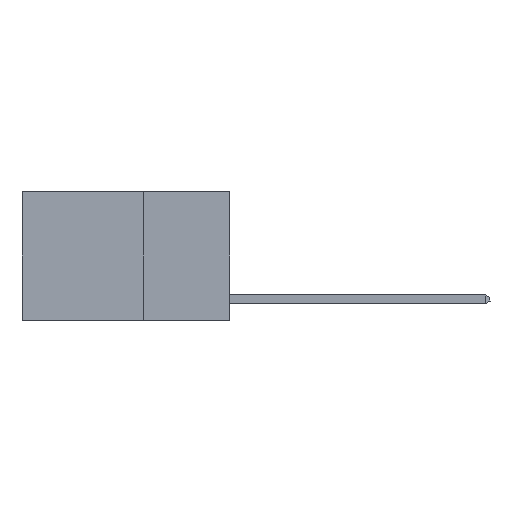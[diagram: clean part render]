
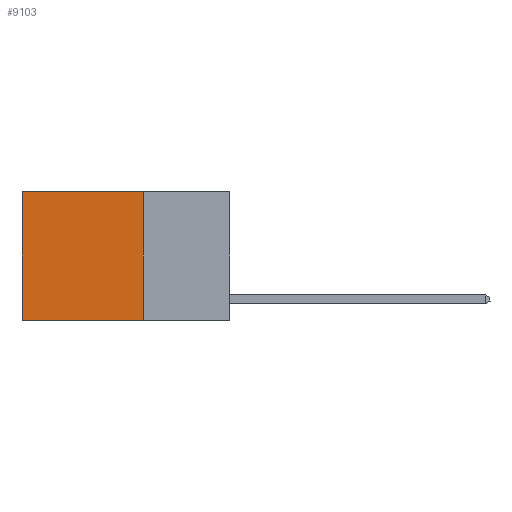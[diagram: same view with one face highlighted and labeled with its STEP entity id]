
A CAD part, left-side view. The second image highlights one B-rep face of the part: STEP entity #9103.
In plain terms, the highlighted planar face has unit normal (-1, 0, 0).
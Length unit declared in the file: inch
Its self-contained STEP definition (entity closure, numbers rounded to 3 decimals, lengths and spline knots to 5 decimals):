
#462 = LINE ( 'NONE', #20775, #28145 ) ;
#796 = ORIENTED_EDGE ( 'NONE', *, *, #27038, .T. ) ;
#2072 = LINE ( 'NONE', #23198, #5950 ) ;
#3762 = AXIS2_PLACEMENT_3D ( 'NONE', #6649, #18120, #24575 ) ;
#4126 = ORIENTED_EDGE ( 'NONE', *, *, #19367, .F. ) ;
#5203 = VECTOR ( 'NONE', #13857, 39.37008 ) ;
#5950 = VECTOR ( 'NONE', #7046, 39.37008 ) ;
#6552 = FACE_OUTER_BOUND ( 'NONE', #15254, .T. ) ;
#6649 = CARTESIAN_POINT ( 'NONE',  ( 0.2625, 0.25, 0. ) ) ;
#7046 = DIRECTION ( 'NONE',  ( 0., 1., 0. ) ) ;
#7233 = EDGE_CURVE ( 'NONE', #23287, #20778, #2072, .T. ) ;
#8322 = EDGE_CURVE ( 'NONE', #26590, #20778, #18528, .T. ) ;
#8589 = CARTESIAN_POINT ( 'NONE',  ( 0.2625, 0.25, 0. ) ) ;
#9103 = ADVANCED_FACE ( 'NONE', ( #6552 ), #14876, .F. ) ;
#11896 = DIRECTION ( 'NONE',  ( 0., 1., 0. ) ) ;
#12887 = LINE ( 'NONE', #8589, #5203 ) ;
#13857 = DIRECTION ( 'NONE',  ( 0., 0., -1. ) ) ;
#14740 = CARTESIAN_POINT ( 'NONE',  ( 0.2625, 0.25, -0.37 ) ) ;
#14876 = PLANE ( 'NONE',  #3762 ) ;
#15254 = EDGE_LOOP ( 'NONE', ( #18761, #21822, #4126, #796 ) ) ;
#15372 = CARTESIAN_POINT ( 'NONE',  ( 0.2625, 0.6, -0.37 ) ) ;
#17946 = CARTESIAN_POINT ( 'NONE',  ( 0.2625, 0.6, 0. ) ) ;
#18120 = DIRECTION ( 'NONE',  ( 1., 0., 0. ) ) ;
#18152 = VECTOR ( 'NONE', #22297, 39.37008 ) ;
#18528 = LINE ( 'NONE', #22395, #18152 ) ;
#18761 = ORIENTED_EDGE ( 'NONE', *, *, #8322, .T. ) ;
#19367 = EDGE_CURVE ( 'NONE', #28267, #23287, #12887, .T. ) ;
#20775 = CARTESIAN_POINT ( 'NONE',  ( 0.2625, 0.25, 0. ) ) ;
#20778 = VERTEX_POINT ( 'NONE', #15372 ) ;
#21822 = ORIENTED_EDGE ( 'NONE', *, *, #7233, .F. ) ;
#22297 = DIRECTION ( 'NONE',  ( 0., 0., -1. ) ) ;
#22395 = CARTESIAN_POINT ( 'NONE',  ( 0.2625, 0.6, 0. ) ) ;
#23198 = CARTESIAN_POINT ( 'NONE',  ( 0.2625, 0.25, -0.37 ) ) ;
#23287 = VERTEX_POINT ( 'NONE', #14740 ) ;
#24575 = DIRECTION ( 'NONE',  ( 0., 0., -1. ) ) ;
#26590 = VERTEX_POINT ( 'NONE', #17946 ) ;
#27038 = EDGE_CURVE ( 'NONE', #28267, #26590, #462, .T. ) ;
#28145 = VECTOR ( 'NONE', #11896, 39.37008 ) ;
#28267 = VERTEX_POINT ( 'NONE', #28612 ) ;
#28612 = CARTESIAN_POINT ( 'NONE',  ( 0.2625, 0.25, 0. ) ) ;
